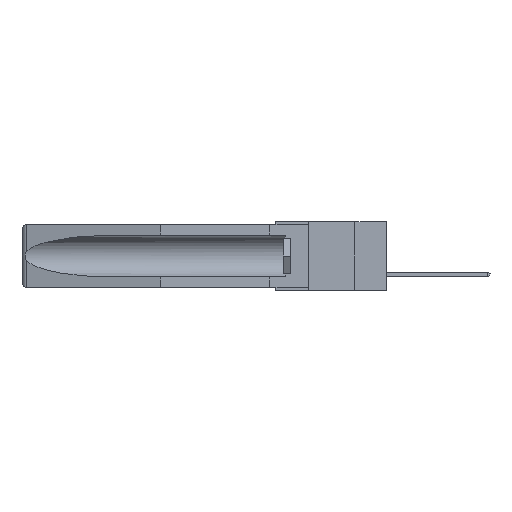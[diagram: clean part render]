
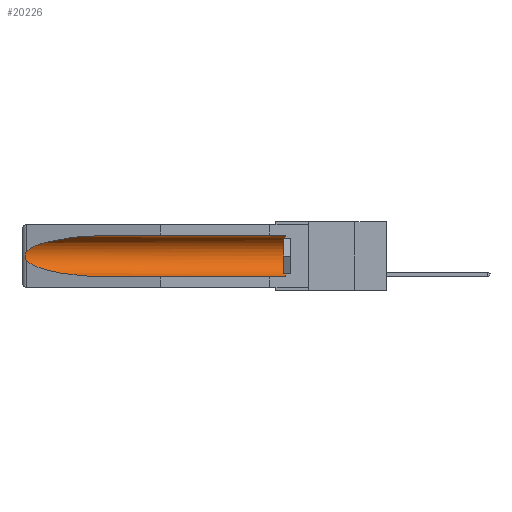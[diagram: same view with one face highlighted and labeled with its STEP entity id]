
A CAD part, left-side view. The second image highlights one B-rep face of the part: STEP entity #20226.
In plain terms, the highlighted cylindrical face has radius 2.857 mm (diameter 5.715 mm), a partial arc.
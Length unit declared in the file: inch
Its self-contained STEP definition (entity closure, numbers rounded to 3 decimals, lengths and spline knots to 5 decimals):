
#256 =( BOUNDED_CURVE ( )  B_SPLINE_CURVE ( 3, ( #17725, #8372, #1005, #17935 ),
 .UNSPECIFIED., .F., .F. ) 
 B_SPLINE_CURVE_WITH_KNOTS ( ( 4, 4 ),
 ( 4.71239, 6.08839 ),
 .UNSPECIFIED. ) 
 CURVE ( )  GEOMETRIC_REPRESENTATION_ITEM ( )  RATIONAL_B_SPLINE_CURVE ( ( 1., 0.848, 0.848, 1. ) ) 
 REPRESENTATION_ITEM ( '' )  );
#1005 = CARTESIAN_POINT ( 'NONE',  ( 0.25451, 1.48313, -0.09465 ) ) ;
#1173 = CARTESIAN_POINT ( 'NONE',  ( 0.26654, 1.53092, -0.15636 ) ) ;
#1404 = VERTEX_POINT ( 'NONE', #28321 ) ;
#1546 = CARTESIAN_POINT ( 'NONE',  ( 0.155, 0.126, -0.059 ) ) ;
#1809 = DIRECTION ( 'NONE',  ( 0., 1., 0. ) ) ;
#1904 = ORIENTED_EDGE ( 'NONE', *, *, #9654, .T. ) ;
#3470 = EDGE_CURVE ( 'NONE', #21935, #13793, #7916, .T. ) ;
#3864 = EDGE_CURVE ( 'NONE', #13793, #1404, #256, .T. ) ;
#5164 = CARTESIAN_POINT ( 'NONE',  ( 0.25451, 1.48313, -0.24835 ) ) ;
#5541 = CARTESIAN_POINT ( 'NONE',  ( 0.26537, 1.52718, -0.19328 ) ) ;
#6464 = CARTESIAN_POINT ( 'NONE',  ( 0.155, 1.07973, -0.284 ) ) ;
#6481 = CARTESIAN_POINT ( 'NONE',  ( 0.155, -0.30754, -0.1715 ) ) ;
#6693 =( BOUNDED_CURVE ( )  B_SPLINE_CURVE ( 3, ( #16931, #5164, #23731, #14244 ),
 .UNSPECIFIED., .F., .T. ) 
 B_SPLINE_CURVE_WITH_KNOTS ( ( 4, 4 ),
 ( 0.1948, 1.5708 ),
 .UNSPECIFIED. ) 
 CURVE ( )  GEOMETRIC_REPRESENTATION_ITEM ( )  RATIONAL_B_SPLINE_CURVE ( ( 1., 0.848, 0.848, 1. ) ) 
 REPRESENTATION_ITEM ( '' )  );
#6773 = FACE_OUTER_BOUND ( 'NONE', #21971, .T. ) ;
#6872 = VERTEX_POINT ( 'NONE', #20824 ) ;
#7916 = LINE ( 'NONE', #8787, #13511 ) ;
#7947 = CARTESIAN_POINT ( 'NONE',  ( 0.2675, 1.53308, -0.16763 ) ) ;
#8372 = CARTESIAN_POINT ( 'NONE',  ( 0.21114, 1.30732, -0.059 ) ) ;
#8696 = DIRECTION ( 'NONE',  ( 0., 0., 1. ) ) ;
#8787 = CARTESIAN_POINT ( 'NONE',  ( 0.155, -0.30754, -0.059 ) ) ;
#9654 = EDGE_CURVE ( 'NONE', #18693, #21935, #10213, .T. ) ;
#10213 = CIRCLE ( 'NONE', #19383, 0.1125 ) ;
#12937 = CARTESIAN_POINT ( 'NONE',  ( 0.155, 1.07973, -0.059 ) ) ;
#13511 = VECTOR ( 'NONE', #15567, 39.37008 ) ;
#13793 = VERTEX_POINT ( 'NONE', #12937 ) ;
#14030 = AXIS2_PLACEMENT_3D ( 'NONE', #6481, #1809, #8696 ) ;
#14244 = CARTESIAN_POINT ( 'NONE',  ( 0.155, 1.07973, -0.284 ) ) ;
#14434 = DIRECTION ( 'NONE',  ( 0., -1., 0. ) ) ;
#15341 = CARTESIAN_POINT ( 'NONE',  ( 0.26655, 1.53094, -0.18657 ) ) ;
#15382 = CYLINDRICAL_SURFACE ( 'NONE', #14030, 0.1125 ) ;
#15567 = DIRECTION ( 'NONE',  ( 0., 1., 0. ) ) ;
#15889 = VERTEX_POINT ( 'NONE', #6464 ) ;
#16483 = DIRECTION ( 'NONE',  ( 0., 0., 1. ) ) ;
#16931 = CARTESIAN_POINT ( 'NONE',  ( 0.26537, 1.52718, -0.19328 ) ) ;
#16993 = CARTESIAN_POINT ( 'NONE',  ( 0.155, 0.126, -0.284 ) ) ;
#17157 = EDGE_CURVE ( 'NONE', #18693, #15889, #30761, .T. ) ;
#17498 = CARTESIAN_POINT ( 'NONE',  ( 0.155, -0.30754, -0.284 ) ) ;
#17597 = CARTESIAN_POINT ( 'NONE',  ( 0.26537, 1.52718, -0.14972 ) ) ;
#17725 = CARTESIAN_POINT ( 'NONE',  ( 0.155, 1.07973, -0.059 ) ) ;
#17935 = CARTESIAN_POINT ( 'NONE',  ( 0.26537, 1.52718, -0.14972 ) ) ;
#18693 = VERTEX_POINT ( 'NONE', #16993 ) ;
#18702 = ORIENTED_EDGE ( 'NONE', *, *, #17157, .F. ) ;
#18773 = CARTESIAN_POINT ( 'NONE',  ( 0.155, 0.126, -0.1715 ) ) ;
#19383 = AXIS2_PLACEMENT_3D ( 'NONE', #18773, #14434, #16483 ) ;
#19722 = ORIENTED_EDGE ( 'NONE', *, *, #22672, .T. ) ;
#19872 = DIRECTION ( 'NONE',  ( 0., 1., 0. ) ) ;
#19974 = CARTESIAN_POINT ( 'NONE',  ( 0.26597, 1.52961, -0.15275 ) ) ;
#20073 = CARTESIAN_POINT ( 'NONE',  ( 0.26597, 1.5296, -0.19026 ) ) ;
#20226 = ADVANCED_FACE ( 'NONE', ( #6773 ), #15382, .F. ) ;
#20824 = CARTESIAN_POINT ( 'NONE',  ( 0.26537, 1.52718, -0.19328 ) ) ;
#21935 = VERTEX_POINT ( 'NONE', #1546 ) ;
#21971 = EDGE_LOOP ( 'NONE', ( #23293, #27267, #19722, #18702, #1904, #28258 ) ) ;
#22672 = EDGE_CURVE ( 'NONE', #6872, #15889, #6693, .T. ) ;
#23293 = ORIENTED_EDGE ( 'NONE', *, *, #3864, .T. ) ;
#23731 = CARTESIAN_POINT ( 'NONE',  ( 0.21114, 1.30732, -0.284 ) ) ;
#24490 = CARTESIAN_POINT ( 'NONE',  ( 0.2675, 1.53308, -0.17534 ) ) ;
#24698 = CARTESIAN_POINT ( 'NONE',  ( 0.2673, 1.53269, -0.17917 ) ) ;
#24787 = CARTESIAN_POINT ( 'NONE',  ( 0.2673, 1.5327, -0.16383 ) ) ;
#25509 = VECTOR ( 'NONE', #19872, 39.37008 ) ;
#25824 = EDGE_CURVE ( 'NONE', #1404, #6872, #28349, .T. ) ;
#27267 = ORIENTED_EDGE ( 'NONE', *, *, #25824, .T. ) ;
#28258 = ORIENTED_EDGE ( 'NONE', *, *, #3470, .T. ) ;
#28321 = CARTESIAN_POINT ( 'NONE',  ( 0.26537, 1.52718, -0.14972 ) ) ;
#28349 = B_SPLINE_CURVE_WITH_KNOTS ( 'NONE', 3,
 ( #17597, #19974, #1173, #24787, #7947, #24490, #24698, #15341, #20073, #5541 ),
 .UNSPECIFIED., .F., .F.,
 ( 4, 2, 2, 2, 4 ),
 ( 0., 0.00029, 0.00058, 0.00087, 0.00117 ),
 .UNSPECIFIED. ) ;
#30761 = LINE ( 'NONE', #17498, #25509 ) ;
